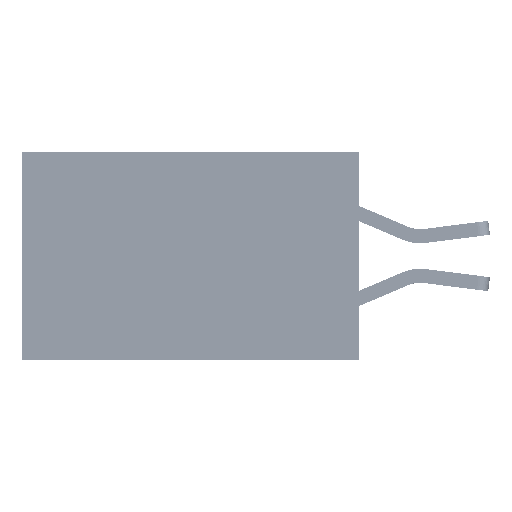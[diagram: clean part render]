
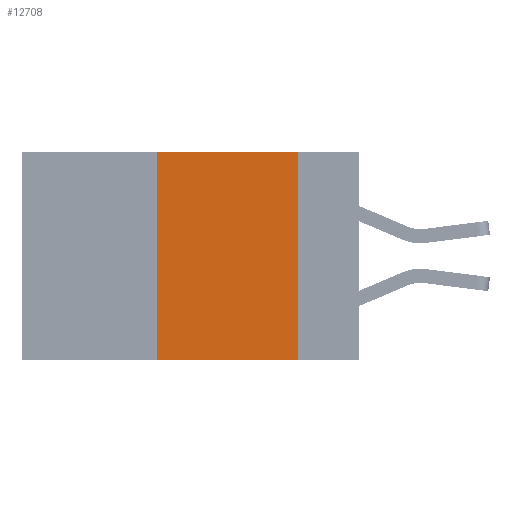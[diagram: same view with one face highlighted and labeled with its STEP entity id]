
A CAD part, left-side view. The second image highlights one B-rep face of the part: STEP entity #12708.
In plain terms, the highlighted planar face has unit normal (-1, 0, 0).
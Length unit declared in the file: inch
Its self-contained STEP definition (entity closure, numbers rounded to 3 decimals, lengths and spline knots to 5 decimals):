
#401 = CARTESIAN_POINT ( 'NONE',  ( 0., 0.36, 0. ) ) ;
#538 = VECTOR ( 'NONE', #34361, 39.37008 ) ;
#965 = VECTOR ( 'NONE', #2747, 39.37008 ) ;
#1157 = VERTEX_POINT ( 'NONE', #38802 ) ;
#1264 = LINE ( 'NONE', #32748, #24264 ) ;
#2747 = DIRECTION ( 'NONE',  ( 0., -1., 0. ) ) ;
#4848 = ORIENTED_EDGE ( 'NONE', *, *, #25726, .T. ) ;
#6796 = CARTESIAN_POINT ( 'NONE',  ( 0., 0.11, 0. ) ) ;
#7842 = DIRECTION ( 'NONE',  ( 0., 0., -1. ) ) ;
#8339 = LINE ( 'NONE', #24619, #965 ) ;
#10367 = VERTEX_POINT ( 'NONE', #6796 ) ;
#11585 = CARTESIAN_POINT ( 'NONE',  ( 0., 0.6, 0. ) ) ;
#11629 = AXIS2_PLACEMENT_3D ( 'NONE', #11585, #14746, #36628 ) ;
#12708 = ADVANCED_FACE ( 'NONE', ( #27940 ), #27138, .F. ) ;
#13046 = VECTOR ( 'NONE', #22306, 39.37008 ) ;
#14746 = DIRECTION ( 'NONE',  ( 1., 0., 0. ) ) ;
#18836 = VERTEX_POINT ( 'NONE', #29702 ) ;
#19010 = EDGE_LOOP ( 'NONE', ( #36432, #25136, #30582, #4848 ) ) ;
#20379 = LINE ( 'NONE', #401, #13046 ) ;
#21739 = CARTESIAN_POINT ( 'NONE',  ( 0., 0.6, 0. ) ) ;
#22306 = DIRECTION ( 'NONE',  ( 0., 0., 1. ) ) ;
#24264 = VECTOR ( 'NONE', #7842, 39.37008 ) ;
#24619 = CARTESIAN_POINT ( 'NONE',  ( 0., 0.6, -0.37 ) ) ;
#25136 = ORIENTED_EDGE ( 'NONE', *, *, #30973, .F. ) ;
#25726 = EDGE_CURVE ( 'NONE', #30910, #18836, #8339, .T. ) ;
#27138 = PLANE ( 'NONE',  #11629 ) ;
#27475 = LINE ( 'NONE', #21739, #538 ) ;
#27819 = EDGE_CURVE ( 'NONE', #30910, #1157, #20379, .T. ) ;
#27940 = FACE_OUTER_BOUND ( 'NONE', #19010, .T. ) ;
#29702 = CARTESIAN_POINT ( 'NONE',  ( 0., 0.11, -0.37 ) ) ;
#30582 = ORIENTED_EDGE ( 'NONE', *, *, #27819, .F. ) ;
#30796 = CARTESIAN_POINT ( 'NONE',  ( 0., 0.36, -0.37 ) ) ;
#30910 = VERTEX_POINT ( 'NONE', #30796 ) ;
#30973 = EDGE_CURVE ( 'NONE', #1157, #10367, #27475, .T. ) ;
#32748 = CARTESIAN_POINT ( 'NONE',  ( 0., 0.11, 0. ) ) ;
#34361 = DIRECTION ( 'NONE',  ( 0., -1., 0. ) ) ;
#36245 = EDGE_CURVE ( 'NONE', #10367, #18836, #1264, .T. ) ;
#36432 = ORIENTED_EDGE ( 'NONE', *, *, #36245, .F. ) ;
#36628 = DIRECTION ( 'NONE',  ( 0., 0., -1. ) ) ;
#38802 = CARTESIAN_POINT ( 'NONE',  ( 0., 0.36, 0. ) ) ;
